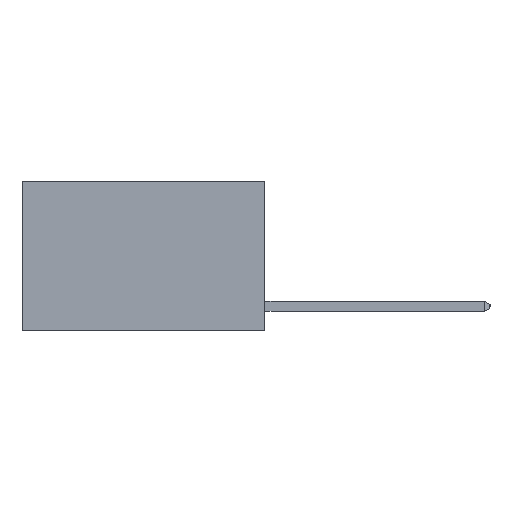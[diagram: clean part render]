
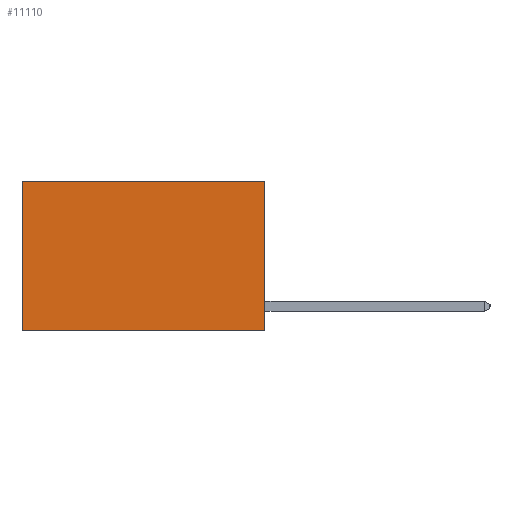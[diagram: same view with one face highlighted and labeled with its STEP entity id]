
A CAD part, left-side view. The second image highlights one B-rep face of the part: STEP entity #11110.
In plain terms, the highlighted planar face has unit normal (-1, 0, 0).
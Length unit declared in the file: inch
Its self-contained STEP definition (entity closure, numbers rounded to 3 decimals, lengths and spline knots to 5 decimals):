
#486 = CARTESIAN_POINT ( 'NONE',  ( 0.2625, 0., 0. ) ) ;
#897 = VERTEX_POINT ( 'NONE', #1819 ) ;
#1197 = EDGE_CURVE ( 'NONE', #7597, #897, #11098, .T. ) ;
#1342 = CARTESIAN_POINT ( 'NONE',  ( 0.2625, 0.6, 0. ) ) ;
#1473 = CARTESIAN_POINT ( 'NONE',  ( 0.2625, 0., 0. ) ) ;
#1502 = VECTOR ( 'NONE', #7421, 39.37008 ) ;
#1671 = LINE ( 'NONE', #6421, #14091 ) ;
#1819 = CARTESIAN_POINT ( 'NONE',  ( 0.2625, 0.6, -0.37 ) ) ;
#2652 = CARTESIAN_POINT ( 'NONE',  ( 0.2625, 0., 0. ) ) ;
#3318 = EDGE_LOOP ( 'NONE', ( #8259, #4653, #9930, #3492 ) ) ;
#3492 = ORIENTED_EDGE ( 'NONE', *, *, #4894, .T. ) ;
#3777 = DIRECTION ( 'NONE',  ( 0., 0., -1. ) ) ;
#4653 = ORIENTED_EDGE ( 'NONE', *, *, #12997, .F. ) ;
#4894 = EDGE_CURVE ( 'NONE', #14281, #7597, #15332, .T. ) ;
#5114 = DIRECTION ( 'NONE',  ( 0., 0., -1. ) ) ;
#6421 = CARTESIAN_POINT ( 'NONE',  ( 0.2625, 0., -0.37 ) ) ;
#6480 = DIRECTION ( 'NONE',  ( 0., 1., 0. ) ) ;
#6828 = DIRECTION ( 'NONE',  ( 0., 1., 0. ) ) ;
#6921 = VECTOR ( 'NONE', #3777, 39.37008 ) ;
#7297 = LINE ( 'NONE', #1473, #6921 ) ;
#7421 = DIRECTION ( 'NONE',  ( 0., 0., -1. ) ) ;
#7588 = CARTESIAN_POINT ( 'NONE',  ( 0.2625, 0.6, 0. ) ) ;
#7597 = VERTEX_POINT ( 'NONE', #7588 ) ;
#8259 = ORIENTED_EDGE ( 'NONE', *, *, #1197, .T. ) ;
#8766 = AXIS2_PLACEMENT_3D ( 'NONE', #2652, #12307, #5114 ) ;
#9065 = CARTESIAN_POINT ( 'NONE',  ( 0.2625, 0., -0.37 ) ) ;
#9905 = PLANE ( 'NONE',  #8766 ) ;
#9930 = ORIENTED_EDGE ( 'NONE', *, *, #14815, .F. ) ;
#11098 = LINE ( 'NONE', #1342, #1502 ) ;
#11110 = ADVANCED_FACE ( 'NONE', ( #13973 ), #9905, .F. ) ;
#11291 = VERTEX_POINT ( 'NONE', #9065 ) ;
#12124 = VECTOR ( 'NONE', #6828, 39.37008 ) ;
#12307 = DIRECTION ( 'NONE',  ( 1., 0., 0. ) ) ;
#12997 = EDGE_CURVE ( 'NONE', #11291, #897, #1671, .T. ) ;
#13973 = FACE_OUTER_BOUND ( 'NONE', #3318, .T. ) ;
#14091 = VECTOR ( 'NONE', #6480, 39.37008 ) ;
#14281 = VERTEX_POINT ( 'NONE', #486 ) ;
#14815 = EDGE_CURVE ( 'NONE', #14281, #11291, #7297, .T. ) ;
#15190 = CARTESIAN_POINT ( 'NONE',  ( 0.2625, 0., 0. ) ) ;
#15332 = LINE ( 'NONE', #15190, #12124 ) ;
